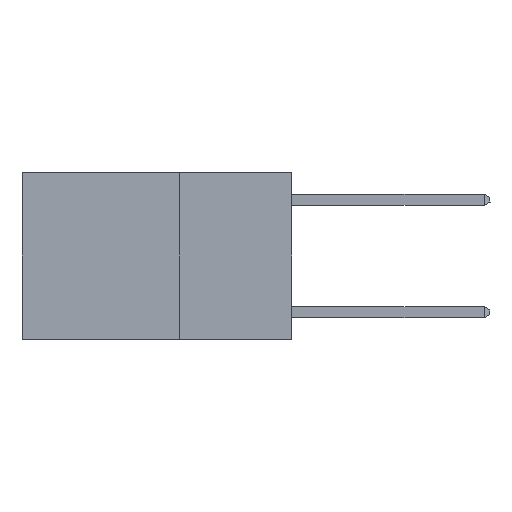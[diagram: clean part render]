
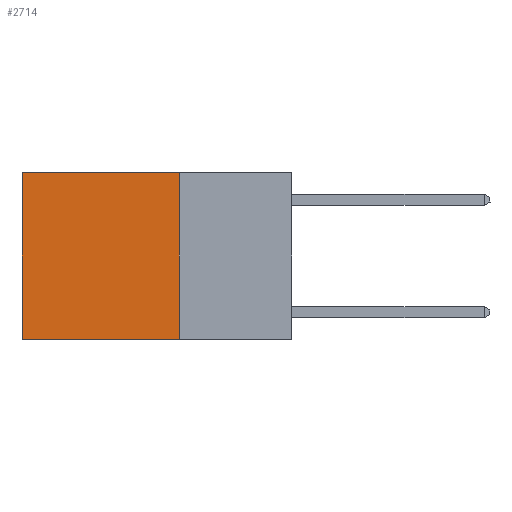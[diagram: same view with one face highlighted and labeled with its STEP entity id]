
A CAD part, left-side view. The second image highlights one B-rep face of the part: STEP entity #2714.
In plain terms, the highlighted planar face has unit normal (-1, 0, 0).
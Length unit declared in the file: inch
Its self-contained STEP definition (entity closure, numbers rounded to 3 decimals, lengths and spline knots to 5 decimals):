
#155 = DIRECTION ( 'NONE',  ( 0., 1., 0. ) ) ;
#243 = VERTEX_POINT ( 'NONE', #8159 ) ;
#271 = VERTEX_POINT ( 'NONE', #1104 ) ;
#1104 = CARTESIAN_POINT ( 'NONE',  ( 0.2625, 0.25, -0.37 ) ) ;
#1812 = CARTESIAN_POINT ( 'NONE',  ( 0.2625, 0.6, 0. ) ) ;
#2156 = VECTOR ( 'NONE', #7059, 39.37008 ) ;
#2167 = AXIS2_PLACEMENT_3D ( 'NONE', #10468, #9425, #11436 ) ;
#2453 = PLANE ( 'NONE',  #2167 ) ;
#2626 = CARTESIAN_POINT ( 'NONE',  ( 0.2625, 0.6, 0. ) ) ;
#2714 = ADVANCED_FACE ( 'NONE', ( #6902 ), #2453, .F. ) ;
#4068 = ORIENTED_EDGE ( 'NONE', *, *, #9991, .F. ) ;
#4093 = ORIENTED_EDGE ( 'NONE', *, *, #7891, .T. ) ;
#4166 = VECTOR ( 'NONE', #155, 39.37008 ) ;
#5105 = VERTEX_POINT ( 'NONE', #5145 ) ;
#5145 = CARTESIAN_POINT ( 'NONE',  ( 0.2625, 0.6, -0.37 ) ) ;
#5619 = EDGE_CURVE ( 'NONE', #243, #9423, #11193, .T. ) ;
#5662 = DIRECTION ( 'NONE',  ( 0., 0., -1. ) ) ;
#5894 = ORIENTED_EDGE ( 'NONE', *, *, #5619, .T. ) ;
#6405 = LINE ( 'NONE', #6883, #2156 ) ;
#6883 = CARTESIAN_POINT ( 'NONE',  ( 0.2625, 0.25, 0. ) ) ;
#6902 = FACE_OUTER_BOUND ( 'NONE', #12916, .T. ) ;
#6949 = VECTOR ( 'NONE', #5662, 39.37008 ) ;
#7059 = DIRECTION ( 'NONE',  ( 0., 0., -1. ) ) ;
#7332 = EDGE_CURVE ( 'NONE', #271, #5105, #10222, .T. ) ;
#7891 = EDGE_CURVE ( 'NONE', #9423, #5105, #11314, .T. ) ;
#8159 = CARTESIAN_POINT ( 'NONE',  ( 0.2625, 0.25, 0. ) ) ;
#9423 = VERTEX_POINT ( 'NONE', #1812 ) ;
#9425 = DIRECTION ( 'NONE',  ( 1., 0., 0. ) ) ;
#9461 = DIRECTION ( 'NONE',  ( 0., 1., 0. ) ) ;
#9991 = EDGE_CURVE ( 'NONE', #243, #271, #6405, .T. ) ;
#10163 = CARTESIAN_POINT ( 'NONE',  ( 0.2625, 0.25, 0. ) ) ;
#10222 = LINE ( 'NONE', #10347, #12724 ) ;
#10347 = CARTESIAN_POINT ( 'NONE',  ( 0.2625, 0.25, -0.37 ) ) ;
#10468 = CARTESIAN_POINT ( 'NONE',  ( 0.2625, 0.25, 0. ) ) ;
#11193 = LINE ( 'NONE', #10163, #4166 ) ;
#11314 = LINE ( 'NONE', #2626, #6949 ) ;
#11436 = DIRECTION ( 'NONE',  ( 0., 0., -1. ) ) ;
#11651 = ORIENTED_EDGE ( 'NONE', *, *, #7332, .F. ) ;
#12724 = VECTOR ( 'NONE', #9461, 39.37008 ) ;
#12916 = EDGE_LOOP ( 'NONE', ( #4093, #11651, #4068, #5894 ) ) ;
